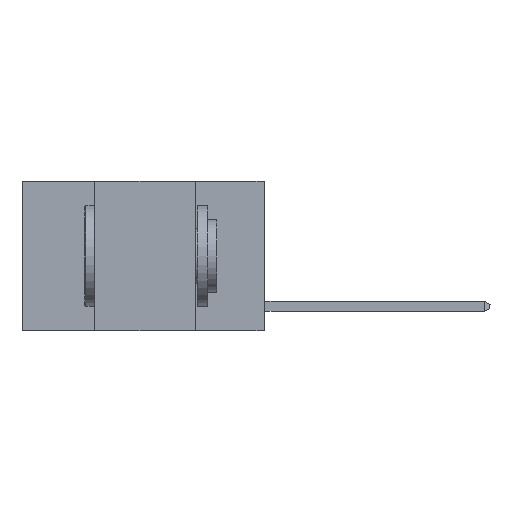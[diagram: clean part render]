
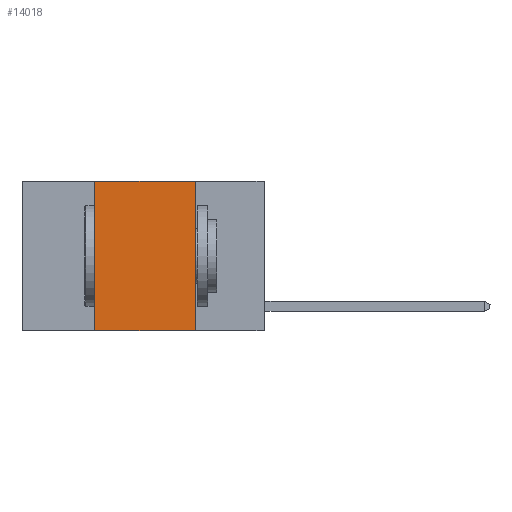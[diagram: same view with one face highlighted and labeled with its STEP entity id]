
A CAD part, left-side view. The second image highlights one B-rep face of the part: STEP entity #14018.
In plain terms, the highlighted planar face has unit normal (-1, 0, 0).
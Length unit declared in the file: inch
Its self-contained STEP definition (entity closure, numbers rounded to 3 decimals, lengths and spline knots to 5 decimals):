
#301 = ORIENTED_EDGE ( 'NONE', *, *, #6498, .F. ) ;
#872 = PLANE ( 'NONE',  #1737 ) ;
#1040 = DIRECTION ( 'NONE',  ( 0., -1., 0. ) ) ;
#1610 = CARTESIAN_POINT ( 'NONE',  ( 0., 0.42, 0. ) ) ;
#1705 = VERTEX_POINT ( 'NONE', #7982 ) ;
#1737 = AXIS2_PLACEMENT_3D ( 'NONE', #7240, #13325, #15887 ) ;
#2355 = EDGE_CURVE ( 'NONE', #4471, #1705, #8740, .T. ) ;
#3741 = EDGE_LOOP ( 'NONE', ( #301, #4833, #11562, #5068 ) ) ;
#4324 = CARTESIAN_POINT ( 'NONE',  ( 0., 0.6, -0.37 ) ) ;
#4471 = VERTEX_POINT ( 'NONE', #1610 ) ;
#4525 = VECTOR ( 'NONE', #14952, 39.37008 ) ;
#4733 = LINE ( 'NONE', #4324, #7674 ) ;
#4823 = FACE_OUTER_BOUND ( 'NONE', #3741, .T. ) ;
#4833 = ORIENTED_EDGE ( 'NONE', *, *, #2355, .F. ) ;
#5068 = ORIENTED_EDGE ( 'NONE', *, *, #8718, .T. ) ;
#5267 = LINE ( 'NONE', #10488, #5451 ) ;
#5451 = VECTOR ( 'NONE', #15482, 39.37008 ) ;
#5773 = VERTEX_POINT ( 'NONE', #7432 ) ;
#6119 = CARTESIAN_POINT ( 'NONE',  ( 0., 0.42, 0. ) ) ;
#6178 = VERTEX_POINT ( 'NONE', #8058 ) ;
#6498 = EDGE_CURVE ( 'NONE', #1705, #6178, #5267, .T. ) ;
#6934 = DIRECTION ( 'NONE',  ( 0., -1., 0. ) ) ;
#7237 = CARTESIAN_POINT ( 'NONE',  ( 0., 0.6, 0. ) ) ;
#7240 = CARTESIAN_POINT ( 'NONE',  ( 0., 0.6, 0. ) ) ;
#7432 = CARTESIAN_POINT ( 'NONE',  ( 0., 0.42, -0.37 ) ) ;
#7674 = VECTOR ( 'NONE', #6934, 39.37008 ) ;
#7982 = CARTESIAN_POINT ( 'NONE',  ( 0., 0.17, 0. ) ) ;
#8058 = CARTESIAN_POINT ( 'NONE',  ( 0., 0.17, -0.37 ) ) ;
#8718 = EDGE_CURVE ( 'NONE', #5773, #6178, #4733, .T. ) ;
#8740 = LINE ( 'NONE', #7237, #12691 ) ;
#9506 = EDGE_CURVE ( 'NONE', #5773, #4471, #15302, .T. ) ;
#10488 = CARTESIAN_POINT ( 'NONE',  ( 0., 0.17, 0. ) ) ;
#11562 = ORIENTED_EDGE ( 'NONE', *, *, #9506, .F. ) ;
#12691 = VECTOR ( 'NONE', #1040, 39.37008 ) ;
#13325 = DIRECTION ( 'NONE',  ( 1., 0., 0. ) ) ;
#14018 = ADVANCED_FACE ( 'NONE', ( #4823 ), #872, .F. ) ;
#14952 = DIRECTION ( 'NONE',  ( 0., 0., 1. ) ) ;
#15302 = LINE ( 'NONE', #6119, #4525 ) ;
#15482 = DIRECTION ( 'NONE',  ( 0., 0., -1. ) ) ;
#15887 = DIRECTION ( 'NONE',  ( 0., 0., -1. ) ) ;
